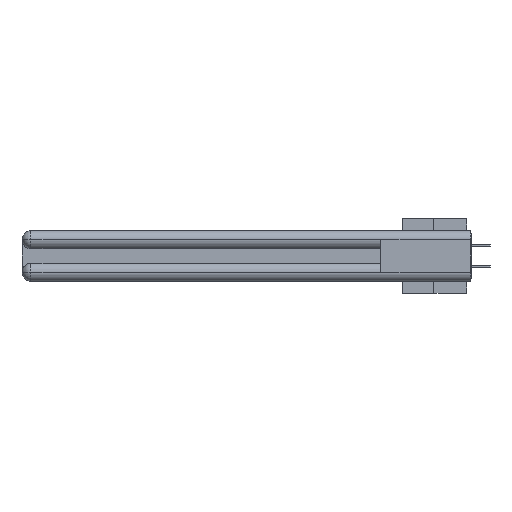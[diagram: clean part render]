
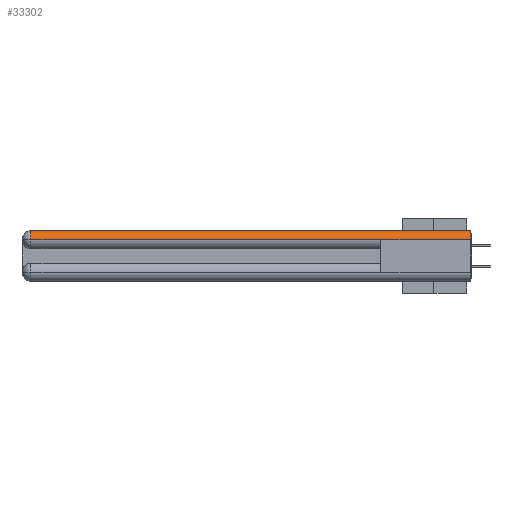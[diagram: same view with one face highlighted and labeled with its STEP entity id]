
A CAD part, left-side view. The second image highlights one B-rep face of the part: STEP entity #33302.
In plain terms, the highlighted cylindrical face has radius 1.562 mm (diameter 3.124 mm), a partial arc.
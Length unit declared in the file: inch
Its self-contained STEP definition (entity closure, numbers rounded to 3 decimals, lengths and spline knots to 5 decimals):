
#348 = EDGE_LOOP ( 'NONE', ( #4760, #11797, #2059, #17105, #19643 ) ) ;
#416 = CYLINDRICAL_SURFACE ( 'NONE', #28836, 0.0615 ) ;
#590 = AXIS2_PLACEMENT_3D ( 'NONE', #6894, #12295, #26555 ) ;
#643 = DIRECTION ( 'NONE',  ( 0., 0., 1. ) ) ;
#2059 = ORIENTED_EDGE ( 'NONE', *, *, #4397, .T. ) ;
#3642 = CARTESIAN_POINT ( 'NONE',  ( 0., 3., -0.0615 ) ) ;
#3797 = EDGE_CURVE ( 'NONE', #35347, #22365, #19901, .T. ) ;
#4397 = EDGE_CURVE ( 'NONE', #22365, #11541, #6193, .T. ) ;
#4760 = ORIENTED_EDGE ( 'NONE', *, *, #13290, .F. ) ;
#4843 = EDGE_CURVE ( 'NONE', #11288, #23375, #16124, .T. ) ;
#5730 = AXIS2_PLACEMENT_3D ( 'NONE', #22515, #33460, #32119 ) ;
#6193 = LINE ( 'NONE', #6425, #34381 ) ;
#6425 = CARTESIAN_POINT ( 'NONE',  ( 0., 3., -0.0615 ) ) ;
#6894 = CARTESIAN_POINT ( 'NONE',  ( 0.0615, 0., -0.0615 ) ) ;
#8521 = VECTOR ( 'NONE', #30729, 39.37008 ) ;
#11288 = VERTEX_POINT ( 'NONE', #16619 ) ;
#11541 = VERTEX_POINT ( 'NONE', #23827 ) ;
#11797 = ORIENTED_EDGE ( 'NONE', *, *, #3797, .T. ) ;
#12295 = DIRECTION ( 'NONE',  ( 0., -1., 0. ) ) ;
#13290 = EDGE_CURVE ( 'NONE', #35347, #11288, #20423, .T. ) ;
#14289 = LINE ( 'NONE', #3642, #26179 ) ;
#15688 = CARTESIAN_POINT ( 'NONE',  ( 0., 2.94, -0.0615 ) ) ;
#16124 = CIRCLE ( 'NONE', #590, 0.0615 ) ;
#16619 = CARTESIAN_POINT ( 'NONE',  ( 0.0615, 0., 0. ) ) ;
#17105 = ORIENTED_EDGE ( 'NONE', *, *, #21229, .F. ) ;
#17371 = CARTESIAN_POINT ( 'NONE',  ( 0.0615, 0., -0.0615 ) ) ;
#19643 = ORIENTED_EDGE ( 'NONE', *, *, #4843, .F. ) ;
#19901 = CIRCLE ( 'NONE', #5730, 0.0615 ) ;
#20395 = CARTESIAN_POINT ( 'NONE',  ( 0.0615, 2.94, 0. ) ) ;
#20423 = LINE ( 'NONE', #25392, #8521 ) ;
#21229 = EDGE_CURVE ( 'NONE', #23375, #11541, #14289, .T. ) ;
#22329 = CARTESIAN_POINT ( 'NONE',  ( 0., 0., -0.0615 ) ) ;
#22365 = VERTEX_POINT ( 'NONE', #15688 ) ;
#22515 = CARTESIAN_POINT ( 'NONE',  ( 0.0615, 2.94, -0.0615 ) ) ;
#23375 = VERTEX_POINT ( 'NONE', #22329 ) ;
#23827 = CARTESIAN_POINT ( 'NONE',  ( 0., 0.6, -0.0615 ) ) ;
#25392 = CARTESIAN_POINT ( 'NONE',  ( 0.0615, 0., 0. ) ) ;
#26179 = VECTOR ( 'NONE', #28889, 39.37008 ) ;
#26555 = DIRECTION ( 'NONE',  ( 1., 0., 0. ) ) ;
#28836 = AXIS2_PLACEMENT_3D ( 'NONE', #17371, #34449, #643 ) ;
#28889 = DIRECTION ( 'NONE',  ( 0., 1., 0. ) ) ;
#29053 = DIRECTION ( 'NONE',  ( 0., -1., 0. ) ) ;
#30729 = DIRECTION ( 'NONE',  ( 0., -1., 0. ) ) ;
#32119 = DIRECTION ( 'NONE',  ( 0., 0., 1. ) ) ;
#33302 = ADVANCED_FACE ( 'NONE', ( #36046 ), #416, .T. ) ;
#33460 = DIRECTION ( 'NONE',  ( 0., -1., 0. ) ) ;
#34381 = VECTOR ( 'NONE', #29053, 39.37008 ) ;
#34449 = DIRECTION ( 'NONE',  ( 0., 1., 0. ) ) ;
#35347 = VERTEX_POINT ( 'NONE', #20395 ) ;
#36046 = FACE_OUTER_BOUND ( 'NONE', #348, .T. ) ;
